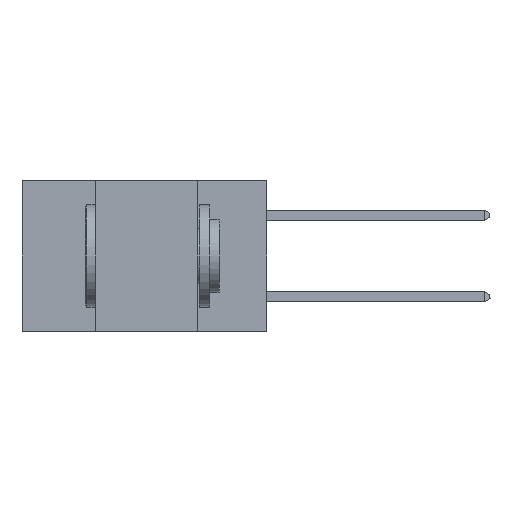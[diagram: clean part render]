
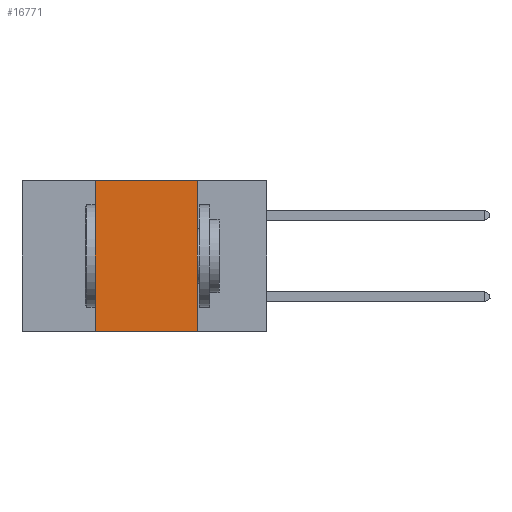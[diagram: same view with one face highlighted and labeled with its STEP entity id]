
A CAD part, left-side view. The second image highlights one B-rep face of the part: STEP entity #16771.
In plain terms, the highlighted planar face has unit normal (-1, 0, 0).
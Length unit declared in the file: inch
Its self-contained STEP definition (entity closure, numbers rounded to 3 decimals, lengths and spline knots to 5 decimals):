
#274 = EDGE_LOOP ( 'NONE', ( #14936, #12766, #10235, #21323 ) ) ;
#1034 = VERTEX_POINT ( 'NONE', #13918 ) ;
#1700 = CARTESIAN_POINT ( 'NONE',  ( 0., 0.17, 0. ) ) ;
#1904 = FACE_OUTER_BOUND ( 'NONE', #274, .T. ) ;
#3348 = CARTESIAN_POINT ( 'NONE',  ( 0., 0.42, -0.37 ) ) ;
#3478 = DIRECTION ( 'NONE',  ( 0., -1., 0. ) ) ;
#4059 = CARTESIAN_POINT ( 'NONE',  ( 0., 0.42, 0. ) ) ;
#6079 = CARTESIAN_POINT ( 'NONE',  ( 0., 0.6, 0. ) ) ;
#6649 = DIRECTION ( 'NONE',  ( 1., 0., 0. ) ) ;
#8176 = VERTEX_POINT ( 'NONE', #1700 ) ;
#8459 = DIRECTION ( 'NONE',  ( 0., 0., -1. ) ) ;
#8529 = CARTESIAN_POINT ( 'NONE',  ( 0., 0.6, 0. ) ) ;
#9633 = VECTOR ( 'NONE', #3478, 39.37008 ) ;
#10235 = ORIENTED_EDGE ( 'NONE', *, *, #21402, .F. ) ;
#11119 = DIRECTION ( 'NONE',  ( 0., 0., 1. ) ) ;
#11586 = CARTESIAN_POINT ( 'NONE',  ( 0., 0.17, -0.37 ) ) ;
#11871 = LINE ( 'NONE', #6079, #18155 ) ;
#12766 = ORIENTED_EDGE ( 'NONE', *, *, #15032, .F. ) ;
#13120 = VERTEX_POINT ( 'NONE', #3348 ) ;
#13270 = DIRECTION ( 'NONE',  ( 0., 0., -1. ) ) ;
#13901 = LINE ( 'NONE', #4059, #21285 ) ;
#13918 = CARTESIAN_POINT ( 'NONE',  ( 0., 0.42, 0. ) ) ;
#14936 = ORIENTED_EDGE ( 'NONE', *, *, #21014, .F. ) ;
#14993 = DIRECTION ( 'NONE',  ( 0., -1., 0. ) ) ;
#15032 = EDGE_CURVE ( 'NONE', #1034, #8176, #11871, .T. ) ;
#15168 = EDGE_CURVE ( 'NONE', #13120, #15613, #15965, .T. ) ;
#15428 = CARTESIAN_POINT ( 'NONE',  ( 0., 0.17, 0. ) ) ;
#15613 = VERTEX_POINT ( 'NONE', #11586 ) ;
#15965 = LINE ( 'NONE', #20945, #9633 ) ;
#16771 = ADVANCED_FACE ( 'NONE', ( #1904 ), #17300, .F. ) ;
#17218 = LINE ( 'NONE', #15428, #18311 ) ;
#17300 = PLANE ( 'NONE',  #18019 ) ;
#18019 = AXIS2_PLACEMENT_3D ( 'NONE', #8529, #6649, #8459 ) ;
#18155 = VECTOR ( 'NONE', #14993, 39.37008 ) ;
#18311 = VECTOR ( 'NONE', #13270, 39.37008 ) ;
#20945 = CARTESIAN_POINT ( 'NONE',  ( 0., 0.6, -0.37 ) ) ;
#21014 = EDGE_CURVE ( 'NONE', #8176, #15613, #17218, .T. ) ;
#21285 = VECTOR ( 'NONE', #11119, 39.37008 ) ;
#21323 = ORIENTED_EDGE ( 'NONE', *, *, #15168, .T. ) ;
#21402 = EDGE_CURVE ( 'NONE', #13120, #1034, #13901, .T. ) ;
